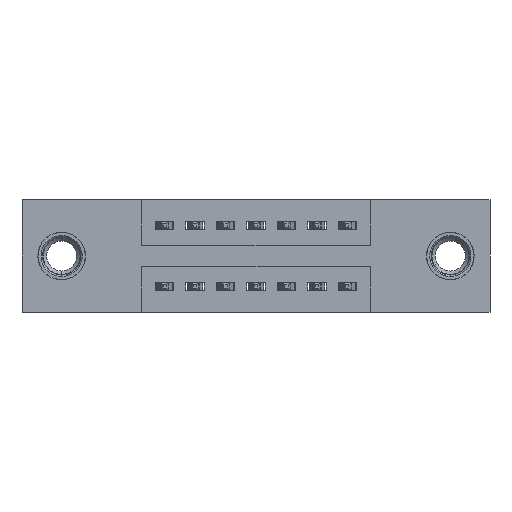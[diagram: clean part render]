
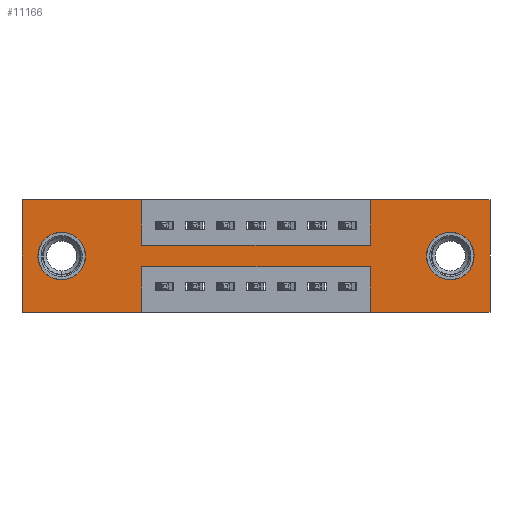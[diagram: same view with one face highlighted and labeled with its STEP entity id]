
A CAD part, front view. The second image highlights one B-rep face of the part: STEP entity #11166.
In plain terms, the highlighted planar face has unit normal (0, -1, 0).
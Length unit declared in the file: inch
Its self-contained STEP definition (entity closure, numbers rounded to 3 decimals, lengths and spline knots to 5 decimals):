
#352 = EDGE_CURVE ( 'NONE', #7877, #10752, #6081, .T. ) ;
#380 = DIRECTION ( 'NONE',  ( 0., 0., -1. ) ) ;
#434 = CARTESIAN_POINT ( 'NONE',  ( 1.405, 0., -0.185 ) ) ;
#624 = FACE_BOUND ( 'NONE', #6827, .T. ) ;
#762 = VECTOR ( 'NONE', #2745, 39.37008 ) ;
#814 = VERTEX_POINT ( 'NONE', #7093 ) ;
#822 = VERTEX_POINT ( 'NONE', #7112 ) ;
#972 = AXIS2_PLACEMENT_3D ( 'NONE', #434, #6632, #1344 ) ;
#1041 = LINE ( 'NONE', #4521, #762 ) ;
#1108 = VERTEX_POINT ( 'NONE', #1162 ) ;
#1129 = DIRECTION ( 'NONE',  ( -1., 0., 0. ) ) ;
#1162 = CARTESIAN_POINT ( 'NONE',  ( 0.13, 0., -0.263 ) ) ;
#1344 = DIRECTION ( 'NONE',  ( 0., 0., -1. ) ) ;
#1384 = DIRECTION ( 'NONE',  ( 0., 0., 1. ) ) ;
#1399 = DIRECTION ( 'NONE',  ( 0., 1., 0. ) ) ;
#1410 = CARTESIAN_POINT ( 'NONE',  ( 0.13, 0., -0.185 ) ) ;
#1531 = LINE ( 'NONE', #8568, #5990 ) ;
#1589 = CARTESIAN_POINT ( 'NONE',  ( 1.1425, 0., 0. ) ) ;
#1596 = CARTESIAN_POINT ( 'NONE',  ( 1.535, 0., 0. ) ) ;
#1638 = DIRECTION ( 'NONE',  ( 0., 0., -1. ) ) ;
#1639 = AXIS2_PLACEMENT_3D ( 'NONE', #10955, #5747, #380 ) ;
#1695 = VERTEX_POINT ( 'NONE', #8376 ) ;
#1953 = CARTESIAN_POINT ( 'NONE',  ( 1.405, 0., -0.263 ) ) ;
#2065 = VERTEX_POINT ( 'NONE', #5921 ) ;
#2208 = DIRECTION ( 'NONE',  ( 0., -1., 0. ) ) ;
#2339 = LINE ( 'NONE', #9119, #9131 ) ;
#2386 = CARTESIAN_POINT ( 'NONE',  ( 0.3925, 0., -0.37 ) ) ;
#2473 = EDGE_CURVE ( 'NONE', #2065, #6276, #10576, .T. ) ;
#2680 = EDGE_CURVE ( 'NONE', #1108, #814, #4041, .T. ) ;
#2745 = DIRECTION ( 'NONE',  ( 0., 0., -1. ) ) ;
#2950 = DIRECTION ( 'NONE',  ( 1., 0., 0. ) ) ;
#2962 = CARTESIAN_POINT ( 'NONE',  ( 0., 0., 0. ) ) ;
#3123 = VERTEX_POINT ( 'NONE', #2386 ) ;
#3163 = PLANE ( 'NONE',  #10625 ) ;
#3507 = VERTEX_POINT ( 'NONE', #9467 ) ;
#3693 = VERTEX_POINT ( 'NONE', #7310 ) ;
#3839 = VECTOR ( 'NONE', #7327, 39.37008 ) ;
#3940 = CARTESIAN_POINT ( 'NONE',  ( 0., 0., -0.37 ) ) ;
#4041 = CIRCLE ( 'NONE', #6687, 0.078 ) ;
#4042 = EDGE_CURVE ( 'NONE', #3693, #11181, #10935, .T. ) ;
#4072 = DIRECTION ( 'NONE',  ( 1., 0., 0. ) ) ;
#4100 = DIRECTION ( 'NONE',  ( 0., 0., -1. ) ) ;
#4157 = DIRECTION ( 'NONE',  ( 1., 0., 0. ) ) ;
#4187 = CARTESIAN_POINT ( 'NONE',  ( 0.3925, 0., -0.15 ) ) ;
#4243 = VERTEX_POINT ( 'NONE', #1953 ) ;
#4288 = EDGE_CURVE ( 'NONE', #1695, #7886, #4406, .T. ) ;
#4406 = LINE ( 'NONE', #1596, #4664 ) ;
#4443 = CARTESIAN_POINT ( 'NONE',  ( 1.1425, 0., -0.37 ) ) ;
#4521 = CARTESIAN_POINT ( 'NONE',  ( 0.3925, 0., 0. ) ) ;
#4642 = CARTESIAN_POINT ( 'NONE',  ( 1.535, 0., -0.37 ) ) ;
#4644 = DIRECTION ( 'NONE',  ( 0., 1., 0. ) ) ;
#4664 = VECTOR ( 'NONE', #1638, 39.37008 ) ;
#4750 = CARTESIAN_POINT ( 'NONE',  ( 0.3925, 0., 0. ) ) ;
#5005 = LINE ( 'NONE', #9196, #6728 ) ;
#5097 = EDGE_CURVE ( 'NONE', #11428, #4243, #7243, .T. ) ;
#5113 = EDGE_CURVE ( 'NONE', #10947, #7877, #9663, .T. ) ;
#5145 = VECTOR ( 'NONE', #9590, 39.37008 ) ;
#5330 = CARTESIAN_POINT ( 'NONE',  ( 1.405, 0., -0.107 ) ) ;
#5747 = DIRECTION ( 'NONE',  ( 0., 1., 0. ) ) ;
#5765 = CARTESIAN_POINT ( 'NONE',  ( 0., 0., 0. ) ) ;
#5826 = VECTOR ( 'NONE', #1129, 39.37008 ) ;
#5860 = ORIENTED_EDGE ( 'NONE', *, *, #5097, .T. ) ;
#5910 = ORIENTED_EDGE ( 'NONE', *, *, #9646, .T. ) ;
#5921 = CARTESIAN_POINT ( 'NONE',  ( 0., 0., 0. ) ) ;
#5938 = ORIENTED_EDGE ( 'NONE', *, *, #9477, .T. ) ;
#5946 = ORIENTED_EDGE ( 'NONE', *, *, #2680, .T. ) ;
#5957 = ORIENTED_EDGE ( 'NONE', *, *, #11072, .F. ) ;
#5990 = VECTOR ( 'NONE', #9486, 39.37008 ) ;
#5991 = ORIENTED_EDGE ( 'NONE', *, *, #352, .F. ) ;
#6022 = ORIENTED_EDGE ( 'NONE', *, *, #5113, .F. ) ;
#6036 = ORIENTED_EDGE ( 'NONE', *, *, #7988, .F. ) ;
#6041 = ORIENTED_EDGE ( 'NONE', *, *, #4288, .F. ) ;
#6062 = ORIENTED_EDGE ( 'NONE', *, *, #7154, .F. ) ;
#6081 = LINE ( 'NONE', #9074, #5826 ) ;
#6084 = ORIENTED_EDGE ( 'NONE', *, *, #10518, .F. ) ;
#6105 = ORIENTED_EDGE ( 'NONE', *, *, #4042, .F. ) ;
#6133 = LINE ( 'NONE', #5765, #7903 ) ;
#6150 = ORIENTED_EDGE ( 'NONE', *, *, #10036, .F. ) ;
#6159 = ORIENTED_EDGE ( 'NONE', *, *, #2473, .F. ) ;
#6171 = ORIENTED_EDGE ( 'NONE', *, *, #11104, .F. ) ;
#6222 = ORIENTED_EDGE ( 'NONE', *, *, #8226, .F. ) ;
#6276 = VERTEX_POINT ( 'NONE', #4750 ) ;
#6444 = DIRECTION ( 'NONE',  ( 0., 0., -1. ) ) ;
#6582 = AXIS2_PLACEMENT_3D ( 'NONE', #9889, #4644, #10734 ) ;
#6632 = DIRECTION ( 'NONE',  ( 0., 1., 0. ) ) ;
#6687 = AXIS2_PLACEMENT_3D ( 'NONE', #1410, #1399, #1384 ) ;
#6728 = VECTOR ( 'NONE', #10893, 39.37008 ) ;
#6827 = EDGE_LOOP ( 'NONE', ( #5938, #5946 ) ) ;
#6982 = VECTOR ( 'NONE', #9317, 39.37008 ) ;
#7093 = CARTESIAN_POINT ( 'NONE',  ( 0.13, 0., -0.107 ) ) ;
#7112 = CARTESIAN_POINT ( 'NONE',  ( 0., 0., -0.37 ) ) ;
#7154 = EDGE_CURVE ( 'NONE', #3507, #1695, #6133, .T. ) ;
#7243 = CIRCLE ( 'NONE', #972, 0.078 ) ;
#7310 = CARTESIAN_POINT ( 'NONE',  ( 0.3925, 0., -0.15 ) ) ;
#7327 = DIRECTION ( 'NONE',  ( -1., 0., 0. ) ) ;
#7411 = LINE ( 'NONE', #1589, #5145 ) ;
#7436 = CARTESIAN_POINT ( 'NONE',  ( 0.3925, 0., -0.22 ) ) ;
#7496 = CARTESIAN_POINT ( 'NONE',  ( 0., 0., -0.37 ) ) ;
#7497 = CARTESIAN_POINT ( 'NONE',  ( 1.1425, 0., -0.37 ) ) ;
#7541 = CIRCLE ( 'NONE', #1639, 0.078 ) ;
#7679 = FACE_OUTER_BOUND ( 'NONE', #8173, .T. ) ;
#7877 = VERTEX_POINT ( 'NONE', #10733 ) ;
#7886 = VERTEX_POINT ( 'NONE', #4642 ) ;
#7903 = VECTOR ( 'NONE', #4072, 39.37008 ) ;
#7965 = FACE_BOUND ( 'NONE', #8625, .T. ) ;
#7988 = EDGE_CURVE ( 'NONE', #7886, #10947, #8460, .T. ) ;
#8173 = EDGE_LOOP ( 'NONE', ( #5957, #5991, #6022, #6036, #6041, #6062, #6084, #6105, #6150, #6159, #6171, #6222 ) ) ;
#8226 = EDGE_CURVE ( 'NONE', #3123, #822, #1531, .T. ) ;
#8376 = CARTESIAN_POINT ( 'NONE',  ( 1.535, 0., 0. ) ) ;
#8460 = LINE ( 'NONE', #3940, #3839 ) ;
#8461 = CARTESIAN_POINT ( 'NONE',  ( 1.1425, 0., -0.15 ) ) ;
#8568 = CARTESIAN_POINT ( 'NONE',  ( 0., 0., -0.37 ) ) ;
#8625 = EDGE_LOOP ( 'NONE', ( #5860, #5910 ) ) ;
#8989 = CIRCLE ( 'NONE', #6582, 0.078 ) ;
#9074 = CARTESIAN_POINT ( 'NONE',  ( 0.3925, 0., -0.22 ) ) ;
#9119 = CARTESIAN_POINT ( 'NONE',  ( 0.3925, 0., -0.37 ) ) ;
#9131 = VECTOR ( 'NONE', #6444, 39.37008 ) ;
#9196 = CARTESIAN_POINT ( 'NONE',  ( 0., 0., 0. ) ) ;
#9317 = DIRECTION ( 'NONE',  ( 0., 0., 1. ) ) ;
#9467 = CARTESIAN_POINT ( 'NONE',  ( 1.1425, 0., 0. ) ) ;
#9477 = EDGE_CURVE ( 'NONE', #814, #1108, #8989, .T. ) ;
#9486 = DIRECTION ( 'NONE',  ( -1., 0., 0. ) ) ;
#9590 = DIRECTION ( 'NONE',  ( 0., 0., 1. ) ) ;
#9646 = EDGE_CURVE ( 'NONE', #4243, #11428, #7541, .T. ) ;
#9663 = LINE ( 'NONE', #7497, #6982 ) ;
#9889 = CARTESIAN_POINT ( 'NONE',  ( 0.13, 0., -0.185 ) ) ;
#10036 = EDGE_CURVE ( 'NONE', #6276, #3693, #1041, .T. ) ;
#10322 = VECTOR ( 'NONE', #2950, 39.37008 ) ;
#10518 = EDGE_CURVE ( 'NONE', #11181, #3507, #7411, .T. ) ;
#10576 = LINE ( 'NONE', #2962, #10322 ) ;
#10625 = AXIS2_PLACEMENT_3D ( 'NONE', #7496, #2208, #4100 ) ;
#10661 = VECTOR ( 'NONE', #4157, 39.37008 ) ;
#10733 = CARTESIAN_POINT ( 'NONE',  ( 1.1425, 0., -0.22 ) ) ;
#10734 = DIRECTION ( 'NONE',  ( 0., 0., 1. ) ) ;
#10752 = VERTEX_POINT ( 'NONE', #7436 ) ;
#10893 = DIRECTION ( 'NONE',  ( 0., 0., 1. ) ) ;
#10935 = LINE ( 'NONE', #4187, #10661 ) ;
#10947 = VERTEX_POINT ( 'NONE', #4443 ) ;
#10955 = CARTESIAN_POINT ( 'NONE',  ( 1.405, 0., -0.185 ) ) ;
#11072 = EDGE_CURVE ( 'NONE', #10752, #3123, #2339, .T. ) ;
#11104 = EDGE_CURVE ( 'NONE', #822, #2065, #5005, .T. ) ;
#11166 = ADVANCED_FACE ( 'NONE', ( #7965, #624, #7679 ), #3163, .T. ) ;
#11181 = VERTEX_POINT ( 'NONE', #8461 ) ;
#11428 = VERTEX_POINT ( 'NONE', #5330 ) ;
